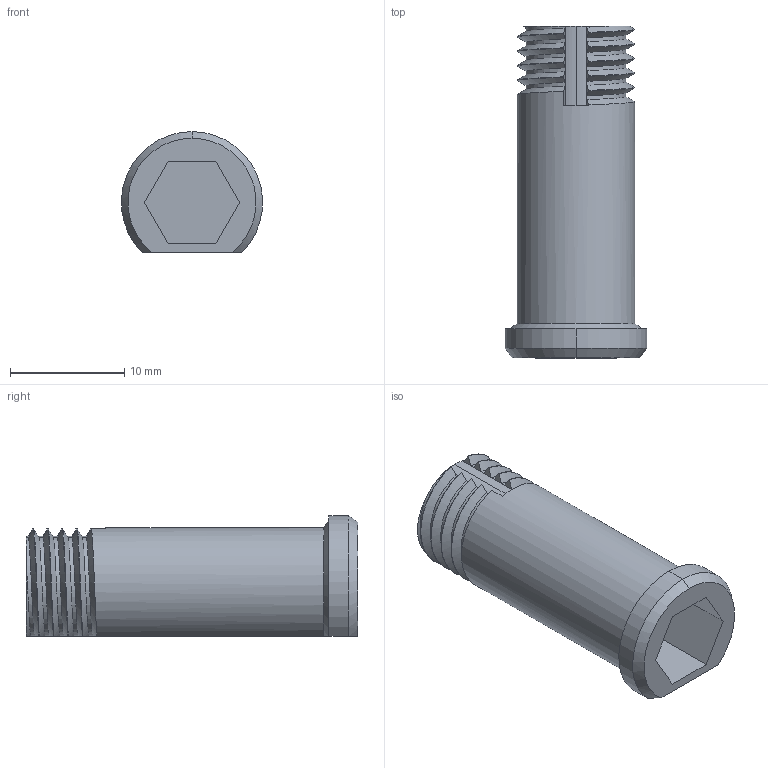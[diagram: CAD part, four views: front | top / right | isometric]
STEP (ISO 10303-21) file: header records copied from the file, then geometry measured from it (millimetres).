
FILE_DESCRIPTION (( 'STEP AP203' ), '1' );
FILE_NAME ('AF-HF-LR-PRT-006-STEP.STEP', '2020-10-04T16:11:24', ( '' ), ( '' ), 'SwSTEP 2.0', 'SolidWorks 2018', '' );
FILE_SCHEMA (( 'CONFIG_CONTROL_DESIGN' ));
Length unit declared in the file: inch
Products named in the file (1): AF-HF-LR-PRT-006-STEP
Bounding box: 12.36 x 29.06 x 10.57 mm (x, y, z)
Volume: 1831.3 mm3; surface area: 1504.1 mm2
Topology: 1 solids, 1 shells, 87 faces, 235 edges, 151 vertices
Faces by surface type: plane 38, bspline 32, cylinder 14, cone 3
Entity records: 8492 total; most frequent: CARTESIAN_POINT 6653, ORIENTED_EDGE 470, DIRECTION 249, EDGE_CURVE 235, VERTEX_POINT 151, VECTOR 111, LINE 111, EDGE_LOOP 88
